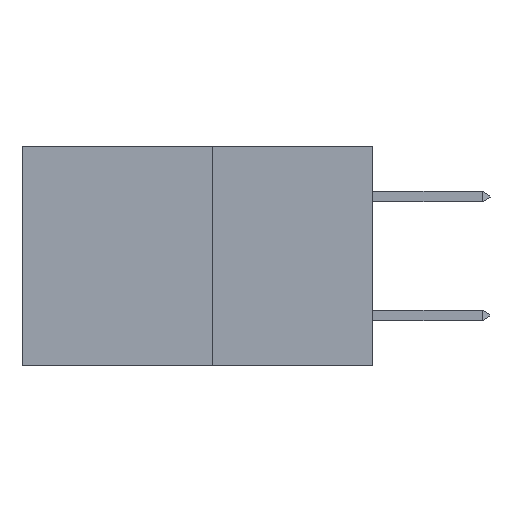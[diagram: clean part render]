
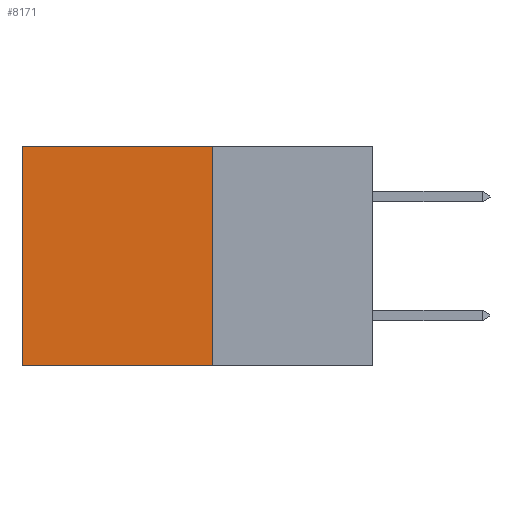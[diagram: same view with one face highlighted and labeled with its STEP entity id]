
A CAD part, left-side view. The second image highlights one B-rep face of the part: STEP entity #8171.
In plain terms, the highlighted planar face has unit normal (-1, 0, 0).
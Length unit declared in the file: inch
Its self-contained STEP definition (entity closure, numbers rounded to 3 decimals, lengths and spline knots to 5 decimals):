
#111 = LINE ( 'NONE', #2792, #2306 ) ;
#281 = DIRECTION ( 'NONE',  ( 1., 0., 0. ) ) ;
#986 = EDGE_CURVE ( 'NONE', #6267, #3918, #9995, .T. ) ;
#1133 = DIRECTION ( 'NONE',  ( 0., 0., -1. ) ) ;
#1253 = CARTESIAN_POINT ( 'NONE',  ( 0.277, 0.27, 0. ) ) ;
#1773 = LINE ( 'NONE', #7358, #5790 ) ;
#2306 = VECTOR ( 'NONE', #1133, 39.37008 ) ;
#2364 = CARTESIAN_POINT ( 'NONE',  ( 0.277, 0.27, -0.37 ) ) ;
#2792 = CARTESIAN_POINT ( 'NONE',  ( 0.277, 0.59, -0.37 ) ) ;
#3070 = AXIS2_PLACEMENT_3D ( 'NONE', #9753, #281, #5926 ) ;
#3640 = ORIENTED_EDGE ( 'NONE', *, *, #5481, .F. ) ;
#3803 = CARTESIAN_POINT ( 'NONE',  ( 0.277, 0.59, -0.37 ) ) ;
#3918 = VERTEX_POINT ( 'NONE', #2364 ) ;
#4015 = EDGE_LOOP ( 'NONE', ( #10113, #3640, #5007, #8827 ) ) ;
#4050 = VECTOR ( 'NONE', #8027, 39.37008 ) ;
#4350 = PLANE ( 'NONE',  #3070 ) ;
#4894 = DIRECTION ( 'NONE',  ( 0., 1., 0. ) ) ;
#4924 = FACE_OUTER_BOUND ( 'NONE', #4015, .T. ) ;
#5007 = ORIENTED_EDGE ( 'NONE', *, *, #986, .F. ) ;
#5481 = EDGE_CURVE ( 'NONE', #3918, #6999, #5955, .T. ) ;
#5608 = CARTESIAN_POINT ( 'NONE',  ( 0.277, 0.27, -0.37 ) ) ;
#5705 = CARTESIAN_POINT ( 'NONE',  ( 0.277, 0.27, -0.37 ) ) ;
#5790 = VECTOR ( 'NONE', #9640, 39.37008 ) ;
#5926 = DIRECTION ( 'NONE',  ( 0., 0., -1. ) ) ;
#5955 = LINE ( 'NONE', #5705, #9798 ) ;
#6031 = CARTESIAN_POINT ( 'NONE',  ( 0.277, 0.59, 0. ) ) ;
#6267 = VERTEX_POINT ( 'NONE', #1253 ) ;
#6999 = VERTEX_POINT ( 'NONE', #3803 ) ;
#7358 = CARTESIAN_POINT ( 'NONE',  ( 0.277, 0.27, 0. ) ) ;
#8027 = DIRECTION ( 'NONE',  ( 0., 0., -1. ) ) ;
#8171 = ADVANCED_FACE ( 'NONE', ( #4924 ), #4350, .F. ) ;
#8231 = EDGE_CURVE ( 'NONE', #8275, #6999, #111, .T. ) ;
#8275 = VERTEX_POINT ( 'NONE', #6031 ) ;
#8717 = EDGE_CURVE ( 'NONE', #6267, #8275, #1773, .T. ) ;
#8827 = ORIENTED_EDGE ( 'NONE', *, *, #8717, .T. ) ;
#9640 = DIRECTION ( 'NONE',  ( 0., 1., 0. ) ) ;
#9753 = CARTESIAN_POINT ( 'NONE',  ( 0.277, 0.27, -0.37 ) ) ;
#9798 = VECTOR ( 'NONE', #4894, 39.37008 ) ;
#9995 = LINE ( 'NONE', #5608, #4050 ) ;
#10113 = ORIENTED_EDGE ( 'NONE', *, *, #8231, .T. ) ;
